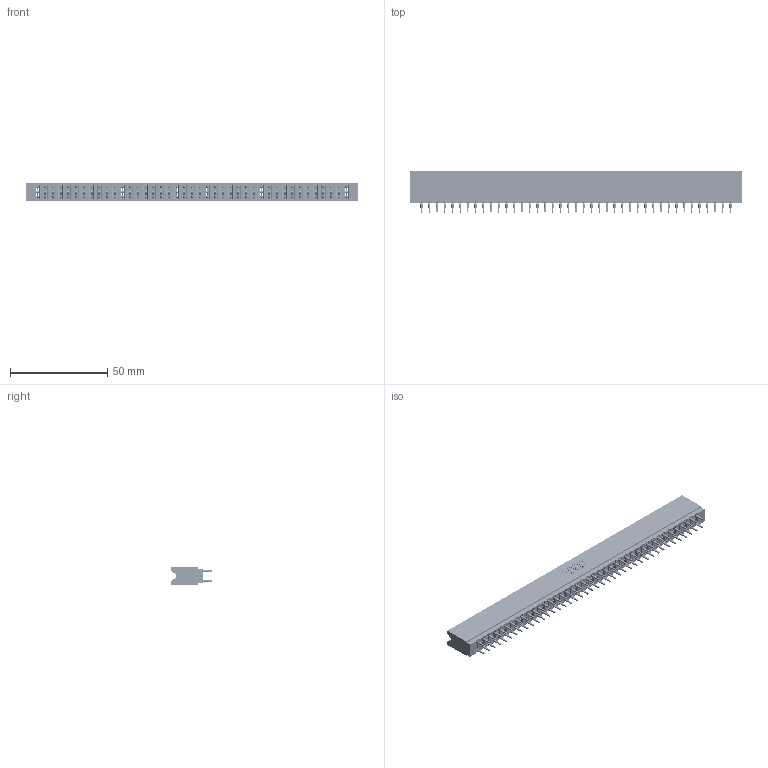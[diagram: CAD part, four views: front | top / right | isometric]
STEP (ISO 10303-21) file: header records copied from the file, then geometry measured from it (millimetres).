
FILE_DESCRIPTION (( 'STEP AP203' ), '1' );
FILE_NAME ('737-082-560-206.STEP', '2026-03-06T02:15:43', ( '' ), ( '' ), 'SwSTEP 2.0', 'SolidWorks 2023', '' );
FILE_SCHEMA (( 'CONFIG_CONTROL_DESIGN' ));
Length unit declared in the file: millimetre
Products named in the file (3): 737-082-560-206; 745-292-001_560; 737 Part_Insulator Option - 06
Assembly tree (83 placements, depth 2):
  737-082-560-206
    737 Part_Insulator Option - 06
    745-292-001_560  x82
Bounding box: 170.33 x 21.22 x 8.89 mm (x, y, z)
Volume: 17063.5 mm3; surface area: 26608.3 mm2
Topology: 83 solids, 83 shells, 8213 faces, 22479 edges, 14274 vertices
Faces by surface type: plane 4278, cylinder 1803, bspline 1640, torus 492
Entity records: 70824 total; most frequent: CARTESIAN_POINT 12800, ORIENTED_EDGE 12234, DIRECTION 10683, EDGE_CURVE 6117, VECTOR 5681, LINE 5681, VERTEX_POINT 3906, AXIS2_PLACEMENT_3D 2501
